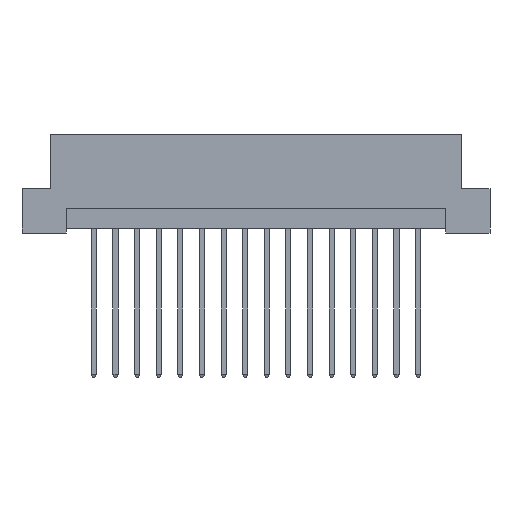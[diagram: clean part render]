
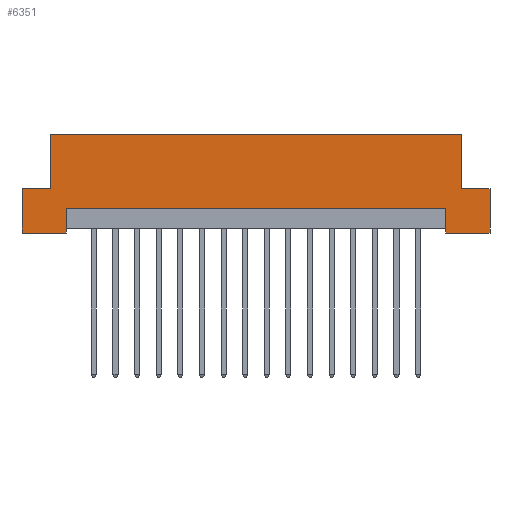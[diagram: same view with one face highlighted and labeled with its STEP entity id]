
A CAD part, front view. The second image highlights one B-rep face of the part: STEP entity #6351.
In plain terms, the highlighted planar face has unit normal (0, -1, 0).
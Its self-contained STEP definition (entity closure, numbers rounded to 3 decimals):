
#6 = VECTOR ( 'NONE', #5061, 1000. ) ;
#77 = CARTESIAN_POINT ( 'NONE',  ( -27.5, 0., 0. ) ) ;
#137 = ORIENTED_EDGE ( 'NONE', *, *, #7501, .F. ) ;
#200 = LINE ( 'NONE', #2445, #9513 ) ;
#229 = EDGE_CURVE ( 'NONE', #3046, #2238, #7919, .T. ) ;
#494 = CARTESIAN_POINT ( 'NONE',  ( 27.5, 0., 0. ) ) ;
#522 = DIRECTION ( 'NONE',  ( 0., 0., 1. ) ) ;
#619 = VERTEX_POINT ( 'NONE', #8490 ) ;
#714 = ORIENTED_EDGE ( 'NONE', *, *, #1491, .T. ) ;
#723 = CARTESIAN_POINT ( 'NONE',  ( 27.5, 0., 5.2 ) ) ;
#734 = LINE ( 'NONE', #3942, #4885 ) ;
#764 = ORIENTED_EDGE ( 'NONE', *, *, #3548, .F. ) ;
#780 = EDGE_CURVE ( 'NONE', #5115, #3759, #6626, .T. ) ;
#883 = EDGE_CURVE ( 'NONE', #4292, #5115, #7331, .T. ) ;
#973 = DIRECTION ( 'NONE',  ( 1., 0., 0. ) ) ;
#986 = DIRECTION ( 'NONE',  ( 0., 0., -1. ) ) ;
#1029 = CARTESIAN_POINT ( 'NONE',  ( -22.3, 0., 2.9 ) ) ;
#1075 = CARTESIAN_POINT ( 'NONE',  ( -24.2, 0., 5.2 ) ) ;
#1148 = LINE ( 'NONE', #5986, #9514 ) ;
#1216 = ORIENTED_EDGE ( 'NONE', *, *, #2653, .F. ) ;
#1266 = ORIENTED_EDGE ( 'NONE', *, *, #2776, .F. ) ;
#1402 = LINE ( 'NONE', #2987, #2947 ) ;
#1491 = EDGE_CURVE ( 'NONE', #3046, #8391, #8708, .T. ) ;
#1845 = CARTESIAN_POINT ( 'NONE',  ( -27.5, 0., 0. ) ) ;
#1857 = CARTESIAN_POINT ( 'NONE',  ( -27.5, 0., 11.6 ) ) ;
#2238 = VERTEX_POINT ( 'NONE', #1029 ) ;
#2239 = ORIENTED_EDGE ( 'NONE', *, *, #229, .F. ) ;
#2244 = CARTESIAN_POINT ( 'NONE',  ( 22.3, 0., 0.5 ) ) ;
#2350 = EDGE_LOOP ( 'NONE', ( #2239, #714, #1266, #137, #10159, #9706, #5085, #10148, #6003, #9444, #1216, #764 ) ) ;
#2365 = VERTEX_POINT ( 'NONE', #7794 ) ;
#2399 = DIRECTION ( 'NONE',  ( 1., 0., 0. ) ) ;
#2445 = CARTESIAN_POINT ( 'NONE',  ( 27.5, 0., 0. ) ) ;
#2630 = VECTOR ( 'NONE', #2399, 1000. ) ;
#2653 = EDGE_CURVE ( 'NONE', #2365, #10204, #734, .T. ) ;
#2736 = CARTESIAN_POINT ( 'NONE',  ( -24.2, 0., 11.6 ) ) ;
#2743 = DIRECTION ( 'NONE',  ( -1., 0., 0. ) ) ;
#2758 = CARTESIAN_POINT ( 'NONE',  ( 24.2, 0., 11.6 ) ) ;
#2776 = EDGE_CURVE ( 'NONE', #6053, #8391, #9048, .T. ) ;
#2788 = AXIS2_PLACEMENT_3D ( 'NONE', #9570, #8777, #5890 ) ;
#2932 = CARTESIAN_POINT ( 'NONE',  ( -22.3, 0., 0.5 ) ) ;
#2947 = VECTOR ( 'NONE', #4671, 1000. ) ;
#2987 = CARTESIAN_POINT ( 'NONE',  ( 24.2, 0., 5.2 ) ) ;
#3046 = VERTEX_POINT ( 'NONE', #4683 ) ;
#3151 = PLANE ( 'NONE',  #2788 ) ;
#3177 = DIRECTION ( 'NONE',  ( -1., 0., 0. ) ) ;
#3429 = EDGE_CURVE ( 'NONE', #10204, #619, #1148, .T. ) ;
#3548 = EDGE_CURVE ( 'NONE', #2238, #2365, #10141, .T. ) ;
#3649 = EDGE_CURVE ( 'NONE', #6342, #3759, #1402, .T. ) ;
#3759 = VERTEX_POINT ( 'NONE', #2758 ) ;
#3942 = CARTESIAN_POINT ( 'NONE',  ( -27.5, 0., 0. ) ) ;
#4044 = DIRECTION ( 'NONE',  ( 1., 0., 0. ) ) ;
#4158 = VECTOR ( 'NONE', #4612, 1000. ) ;
#4268 = DIRECTION ( 'NONE',  ( 0., 0., 1. ) ) ;
#4292 = VERTEX_POINT ( 'NONE', #9628 ) ;
#4401 = CARTESIAN_POINT ( 'NONE',  ( 22.3, 0., 0. ) ) ;
#4612 = DIRECTION ( 'NONE',  ( 0., 0., -1. ) ) ;
#4671 = DIRECTION ( 'NONE',  ( 0., 0., 1. ) ) ;
#4683 = CARTESIAN_POINT ( 'NONE',  ( 22.3, 0., 2.9 ) ) ;
#4885 = VECTOR ( 'NONE', #2743, 1000. ) ;
#5061 = DIRECTION ( 'NONE',  ( -1., 0., 0. ) ) ;
#5085 = ORIENTED_EDGE ( 'NONE', *, *, #780, .F. ) ;
#5115 = VERTEX_POINT ( 'NONE', #2736 ) ;
#5143 = VECTOR ( 'NONE', #4268, 1000. ) ;
#5464 = LINE ( 'NONE', #8245, #6469 ) ;
#5623 = CARTESIAN_POINT ( 'NONE',  ( 24.2, 0., 5.2 ) ) ;
#5890 = DIRECTION ( 'NONE',  ( 0., 0., 1. ) ) ;
#5986 = CARTESIAN_POINT ( 'NONE',  ( -27.5, 0., 0. ) ) ;
#6003 = ORIENTED_EDGE ( 'NONE', *, *, #9627, .F. ) ;
#6053 = VERTEX_POINT ( 'NONE', #494 ) ;
#6283 = CARTESIAN_POINT ( 'NONE',  ( -27.5, 0., 5.2 ) ) ;
#6342 = VERTEX_POINT ( 'NONE', #5623 ) ;
#6351 = ADVANCED_FACE ( 'NONE', ( #7229 ), #3151, .F. ) ;
#6469 = VECTOR ( 'NONE', #4044, 1000. ) ;
#6473 = VECTOR ( 'NONE', #973, 1000. ) ;
#6626 = LINE ( 'NONE', #1857, #6473 ) ;
#6809 = VERTEX_POINT ( 'NONE', #723 ) ;
#7132 = LINE ( 'NONE', #6283, #2630 ) ;
#7221 = VECTOR ( 'NONE', #3177, 1000. ) ;
#7229 = FACE_OUTER_BOUND ( 'NONE', #2350, .T. ) ;
#7331 = LINE ( 'NONE', #1075, #5143 ) ;
#7501 = EDGE_CURVE ( 'NONE', #6809, #6053, #200, .T. ) ;
#7771 = DIRECTION ( 'NONE',  ( 0., 0., -1. ) ) ;
#7794 = CARTESIAN_POINT ( 'NONE',  ( -22.3, 0., 0. ) ) ;
#7919 = LINE ( 'NONE', #9544, #7221 ) ;
#8245 = CARTESIAN_POINT ( 'NONE',  ( 27.5, 0., 5.2 ) ) ;
#8391 = VERTEX_POINT ( 'NONE', #4401 ) ;
#8437 = VECTOR ( 'NONE', #7771, 1000. ) ;
#8490 = CARTESIAN_POINT ( 'NONE',  ( -27.5, 0., 5.2 ) ) ;
#8708 = LINE ( 'NONE', #2244, #4158 ) ;
#8777 = DIRECTION ( 'NONE',  ( 0., 1., 0. ) ) ;
#9048 = LINE ( 'NONE', #1845, #6 ) ;
#9080 = EDGE_CURVE ( 'NONE', #6342, #6809, #5464, .T. ) ;
#9444 = ORIENTED_EDGE ( 'NONE', *, *, #3429, .F. ) ;
#9513 = VECTOR ( 'NONE', #986, 1000. ) ;
#9514 = VECTOR ( 'NONE', #522, 1000. ) ;
#9544 = CARTESIAN_POINT ( 'NONE',  ( 22.3, 0., 2.9 ) ) ;
#9570 = CARTESIAN_POINT ( 'NONE',  ( -27.5, 0., 11.6 ) ) ;
#9627 = EDGE_CURVE ( 'NONE', #619, #4292, #7132, .T. ) ;
#9628 = CARTESIAN_POINT ( 'NONE',  ( -24.2, 0., 5.2 ) ) ;
#9706 = ORIENTED_EDGE ( 'NONE', *, *, #3649, .T. ) ;
#10141 = LINE ( 'NONE', #2932, #8437 ) ;
#10148 = ORIENTED_EDGE ( 'NONE', *, *, #883, .F. ) ;
#10159 = ORIENTED_EDGE ( 'NONE', *, *, #9080, .F. ) ;
#10204 = VERTEX_POINT ( 'NONE', #77 ) ;
